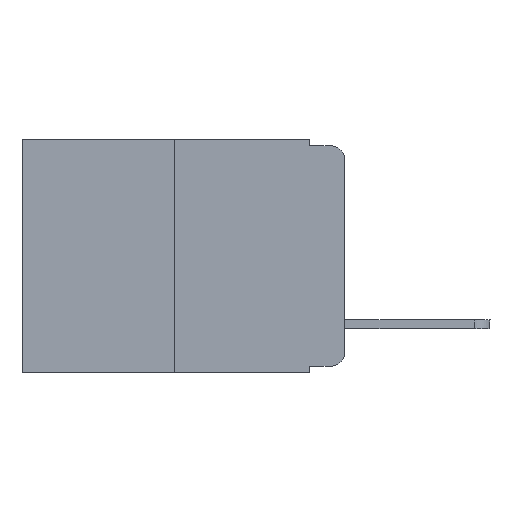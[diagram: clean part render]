
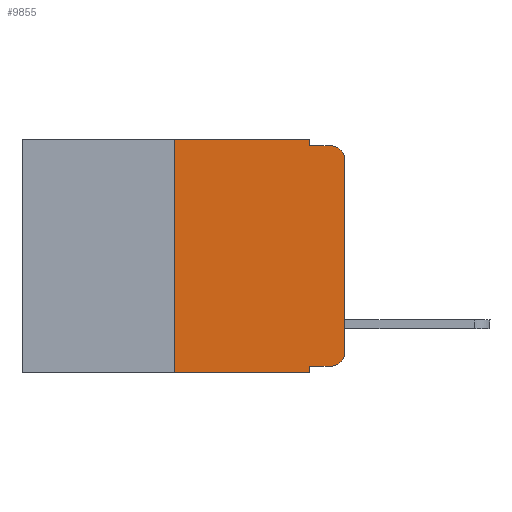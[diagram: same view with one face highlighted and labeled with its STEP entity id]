
A CAD part, left-side view. The second image highlights one B-rep face of the part: STEP entity #9855.
In plain terms, the highlighted planar face has unit normal (-1, 0, 0).
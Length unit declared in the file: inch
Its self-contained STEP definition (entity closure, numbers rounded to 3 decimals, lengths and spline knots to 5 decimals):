
#347 = VECTOR ( 'NONE', #18765, 39.37008 ) ;
#593 = EDGE_CURVE ( 'NONE', #19957, #6503, #14557, .T. ) ;
#769 = DIRECTION ( 'NONE',  ( 0., -1., 0. ) ) ;
#816 = VERTEX_POINT ( 'NONE', #3490 ) ;
#1233 = ORIENTED_EDGE ( 'NONE', *, *, #13690, .T. ) ;
#1306 = CARTESIAN_POINT ( 'NONE',  ( 0., 0., 0. ) ) ;
#1567 = VERTEX_POINT ( 'NONE', #5093 ) ;
#1636 = ORIENTED_EDGE ( 'NONE', *, *, #13796, .T. ) ;
#2115 = EDGE_CURVE ( 'NONE', #18823, #19957, #18980, .T. ) ;
#2543 = VECTOR ( 'NONE', #12452, 39.37008 ) ;
#3372 = CARTESIAN_POINT ( 'NONE',  ( 0., 0.051, 0. ) ) ;
#3381 = ORIENTED_EDGE ( 'NONE', *, *, #10859, .T. ) ;
#3490 = CARTESIAN_POINT ( 'NONE',  ( 0., 0.02, -0.01 ) ) ;
#3501 = CARTESIAN_POINT ( 'NONE',  ( 0., 0., -0.313 ) ) ;
#3558 = CARTESIAN_POINT ( 'NONE',  ( 0., 0.051, -0.01 ) ) ;
#4572 = VERTEX_POINT ( 'NONE', #11416 ) ;
#4791 = DIRECTION ( 'NONE',  ( -1., 0., 0. ) ) ;
#4969 = FACE_OUTER_BOUND ( 'NONE', #11108, .T. ) ;
#5093 = CARTESIAN_POINT ( 'NONE',  ( 0., 0.051, -0.333 ) ) ;
#5514 = CARTESIAN_POINT ( 'NONE',  ( 0., 0.25, 0. ) ) ;
#5733 = DIRECTION ( 'NONE',  ( 0., 0., -1. ) ) ;
#6503 = VERTEX_POINT ( 'NONE', #3558 ) ;
#6702 = LINE ( 'NONE', #3372, #7178 ) ;
#6852 = DIRECTION ( 'NONE',  ( 0., 0., -1. ) ) ;
#6918 = AXIS2_PLACEMENT_3D ( 'NONE', #20985, #18993, #5733 ) ;
#6956 = CARTESIAN_POINT ( 'NONE',  ( 0., 0.473, 0. ) ) ;
#7069 = AXIS2_PLACEMENT_3D ( 'NONE', #6956, #8530, #6852 ) ;
#7149 = CIRCLE ( 'NONE', #12881, 0.02 ) ;
#7159 = CARTESIAN_POINT ( 'NONE',  ( 0., 0.473, 0. ) ) ;
#7178 = VECTOR ( 'NONE', #18838, 39.37008 ) ;
#7763 = VECTOR ( 'NONE', #21347, 39.37008 ) ;
#8530 = DIRECTION ( 'NONE',  ( 1., 0., 0. ) ) ;
#9240 = ORIENTED_EDGE ( 'NONE', *, *, #17342, .T. ) ;
#9637 = VECTOR ( 'NONE', #16680, 39.37008 ) ;
#9792 = LINE ( 'NONE', #1306, #9637 ) ;
#9855 = ADVANCED_FACE ( 'NONE', ( #4969 ), #11664, .F. ) ;
#10126 = CARTESIAN_POINT ( 'NONE',  ( 0., 0.25, 0. ) ) ;
#10468 = CARTESIAN_POINT ( 'NONE',  ( 0., 0.051, -0.01 ) ) ;
#10512 = ORIENTED_EDGE ( 'NONE', *, *, #2115, .F. ) ;
#10683 = DIRECTION ( 'NONE',  ( 0., -1., 0. ) ) ;
#10859 = EDGE_CURVE ( 'NONE', #16226, #4572, #9792, .T. ) ;
#11108 = EDGE_LOOP ( 'NONE', ( #3381, #15830, #20829, #17304, #10512, #13727, #9240, #18554, #1636, #1233 ) ) ;
#11416 = CARTESIAN_POINT ( 'NONE',  ( 0., 0., -0.03 ) ) ;
#11589 = DIRECTION ( 'NONE',  ( 0., 0., -1. ) ) ;
#11664 = PLANE ( 'NONE',  #7069 ) ;
#12364 = LINE ( 'NONE', #10468, #16426 ) ;
#12452 = DIRECTION ( 'NONE',  ( 0., -1., 0. ) ) ;
#12543 = CARTESIAN_POINT ( 'NONE',  ( 0., 0.051, 0. ) ) ;
#12881 = AXIS2_PLACEMENT_3D ( 'NONE', #13163, #4791, #11589 ) ;
#13163 = CARTESIAN_POINT ( 'NONE',  ( 0., 0.02, -0.313 ) ) ;
#13335 = EDGE_CURVE ( 'NONE', #6503, #816, #12364, .T. ) ;
#13365 = VECTOR ( 'NONE', #769, 39.37008 ) ;
#13690 = EDGE_CURVE ( 'NONE', #19948, #16226, #7149, .T. ) ;
#13727 = ORIENTED_EDGE ( 'NONE', *, *, #17679, .F. ) ;
#13769 = CARTESIAN_POINT ( 'NONE',  ( 0., 0.051, -0.343 ) ) ;
#13796 = EDGE_CURVE ( 'NONE', #1567, #19948, #14017, .T. ) ;
#14017 = LINE ( 'NONE', #19129, #2543 ) ;
#14252 = VERTEX_POINT ( 'NONE', #13769 ) ;
#14323 = DIRECTION ( 'NONE',  ( 0., 0., 1. ) ) ;
#14483 = EDGE_CURVE ( 'NONE', #1567, #14252, #6702, .T. ) ;
#14557 = LINE ( 'NONE', #12543, #7763 ) ;
#15830 = ORIENTED_EDGE ( 'NONE', *, *, #17637, .T. ) ;
#16226 = VERTEX_POINT ( 'NONE', #3501 ) ;
#16268 = CARTESIAN_POINT ( 'NONE',  ( 0., 0.051, 0. ) ) ;
#16426 = VECTOR ( 'NONE', #10683, 39.37008 ) ;
#16555 = CIRCLE ( 'NONE', #6918, 0.02 ) ;
#16680 = DIRECTION ( 'NONE',  ( 0., 0., 1. ) ) ;
#17304 = ORIENTED_EDGE ( 'NONE', *, *, #593, .F. ) ;
#17342 = EDGE_CURVE ( 'NONE', #19475, #14252, #21386, .T. ) ;
#17637 = EDGE_CURVE ( 'NONE', #4572, #816, #16555, .T. ) ;
#17679 = EDGE_CURVE ( 'NONE', #19475, #18823, #19211, .T. ) ;
#18554 = ORIENTED_EDGE ( 'NONE', *, *, #14483, .F. ) ;
#18682 = CARTESIAN_POINT ( 'NONE',  ( 0., 0.25, -0.343 ) ) ;
#18765 = DIRECTION ( 'NONE',  ( 0., -1., 0. ) ) ;
#18823 = VERTEX_POINT ( 'NONE', #10126 ) ;
#18833 = CARTESIAN_POINT ( 'NONE',  ( 0., 0.02, -0.333 ) ) ;
#18838 = DIRECTION ( 'NONE',  ( 0., 0., -1. ) ) ;
#18980 = LINE ( 'NONE', #7159, #347 ) ;
#18993 = DIRECTION ( 'NONE',  ( -1., 0., 0. ) ) ;
#19129 = CARTESIAN_POINT ( 'NONE',  ( 0., 0.051, -0.333 ) ) ;
#19211 = LINE ( 'NONE', #5514, #21889 ) ;
#19475 = VERTEX_POINT ( 'NONE', #18682 ) ;
#19948 = VERTEX_POINT ( 'NONE', #18833 ) ;
#19957 = VERTEX_POINT ( 'NONE', #16268 ) ;
#20829 = ORIENTED_EDGE ( 'NONE', *, *, #13335, .F. ) ;
#20922 = CARTESIAN_POINT ( 'NONE',  ( 0., 0.473, -0.343 ) ) ;
#20985 = CARTESIAN_POINT ( 'NONE',  ( 0., 0.02, -0.03 ) ) ;
#21347 = DIRECTION ( 'NONE',  ( 0., 0., -1. ) ) ;
#21386 = LINE ( 'NONE', #20922, #13365 ) ;
#21889 = VECTOR ( 'NONE', #14323, 39.37008 ) ;
